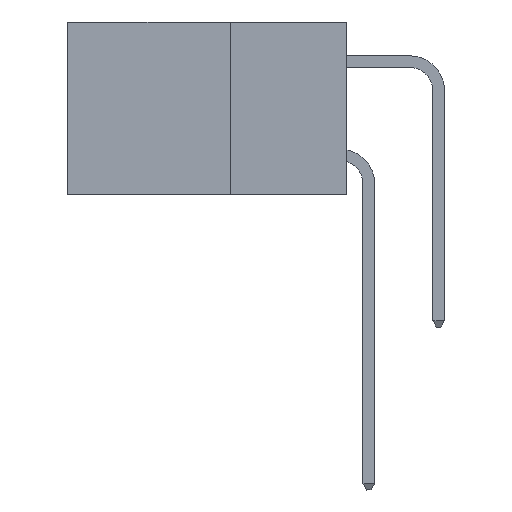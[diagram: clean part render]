
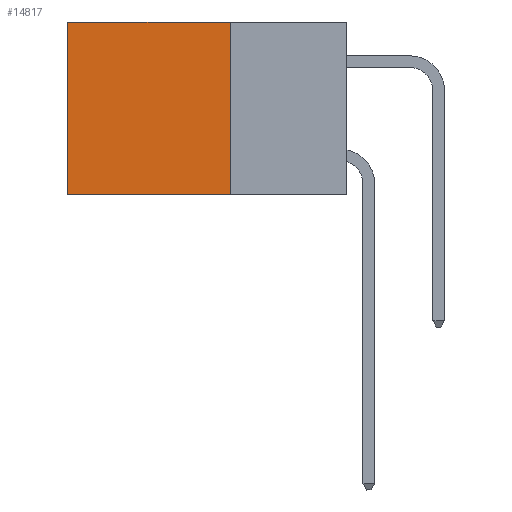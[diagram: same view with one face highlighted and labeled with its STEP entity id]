
A CAD part, left-side view. The second image highlights one B-rep face of the part: STEP entity #14817.
In plain terms, the highlighted planar face has unit normal (-1, 0, 0).
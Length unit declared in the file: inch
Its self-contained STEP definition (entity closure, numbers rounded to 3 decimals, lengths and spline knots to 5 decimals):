
#798 = VERTEX_POINT ( 'NONE', #2575 ) ;
#1419 = CARTESIAN_POINT ( 'NONE',  ( 0.2875, 0.25, 0. ) ) ;
#2573 = EDGE_CURVE ( 'NONE', #14263, #798, #8929, .T. ) ;
#2575 = CARTESIAN_POINT ( 'NONE',  ( 0.2875, 0.25, -0.37 ) ) ;
#2723 = DIRECTION ( 'NONE',  ( 0., 0., -1. ) ) ;
#3031 = AXIS2_PLACEMENT_3D ( 'NONE', #1419, #3892, #10904 ) ;
#3892 = DIRECTION ( 'NONE',  ( 1., 0., 0. ) ) ;
#5406 = ORIENTED_EDGE ( 'NONE', *, *, #8417, .T. ) ;
#5579 = LINE ( 'NONE', #14292, #14750 ) ;
#5768 = LINE ( 'NONE', #6687, #8529 ) ;
#5873 = ORIENTED_EDGE ( 'NONE', *, *, #7576, .T. ) ;
#6007 = VERTEX_POINT ( 'NONE', #6548 ) ;
#6081 = CARTESIAN_POINT ( 'NONE',  ( 0.2875, 0.25, 0. ) ) ;
#6548 = CARTESIAN_POINT ( 'NONE',  ( 0.2875, 0.6, 0. ) ) ;
#6653 = CARTESIAN_POINT ( 'NONE',  ( 0.2875, 0.6, -0.37 ) ) ;
#6687 = CARTESIAN_POINT ( 'NONE',  ( 0.2875, 0.6, 0. ) ) ;
#7576 = EDGE_CURVE ( 'NONE', #14263, #6007, #5579, .T. ) ;
#8216 = FACE_OUTER_BOUND ( 'NONE', #10331, .T. ) ;
#8417 = EDGE_CURVE ( 'NONE', #6007, #11697, #5768, .T. ) ;
#8529 = VECTOR ( 'NONE', #2723, 39.37008 ) ;
#8658 = DIRECTION ( 'NONE',  ( 0., 0., -1. ) ) ;
#8922 = DIRECTION ( 'NONE',  ( 0., 1., 0. ) ) ;
#8929 = LINE ( 'NONE', #6081, #10415 ) ;
#9278 = EDGE_CURVE ( 'NONE', #798, #11697, #13430, .T. ) ;
#9814 = CARTESIAN_POINT ( 'NONE',  ( 0.2875, 0.25, -0.37 ) ) ;
#10331 = EDGE_LOOP ( 'NONE', ( #5406, #12919, #16512, #5873 ) ) ;
#10415 = VECTOR ( 'NONE', #8658, 39.37008 ) ;
#10904 = DIRECTION ( 'NONE',  ( 0., 0., -1. ) ) ;
#11697 = VERTEX_POINT ( 'NONE', #6653 ) ;
#12919 = ORIENTED_EDGE ( 'NONE', *, *, #9278, .F. ) ;
#12993 = VECTOR ( 'NONE', #15174, 39.37008 ) ;
#13430 = LINE ( 'NONE', #9814, #12993 ) ;
#14263 = VERTEX_POINT ( 'NONE', #17493 ) ;
#14292 = CARTESIAN_POINT ( 'NONE',  ( 0.2875, 0.25, 0. ) ) ;
#14750 = VECTOR ( 'NONE', #8922, 39.37008 ) ;
#14778 = PLANE ( 'NONE',  #3031 ) ;
#14817 = ADVANCED_FACE ( 'NONE', ( #8216 ), #14778, .F. ) ;
#15174 = DIRECTION ( 'NONE',  ( 0., 1., 0. ) ) ;
#16512 = ORIENTED_EDGE ( 'NONE', *, *, #2573, .F. ) ;
#17493 = CARTESIAN_POINT ( 'NONE',  ( 0.2875, 0.25, 0. ) ) ;
